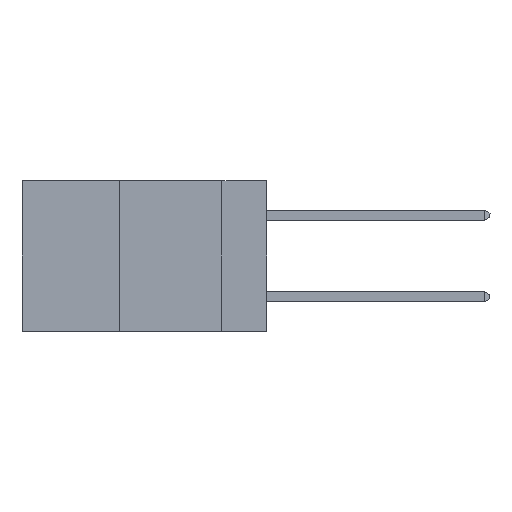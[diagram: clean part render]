
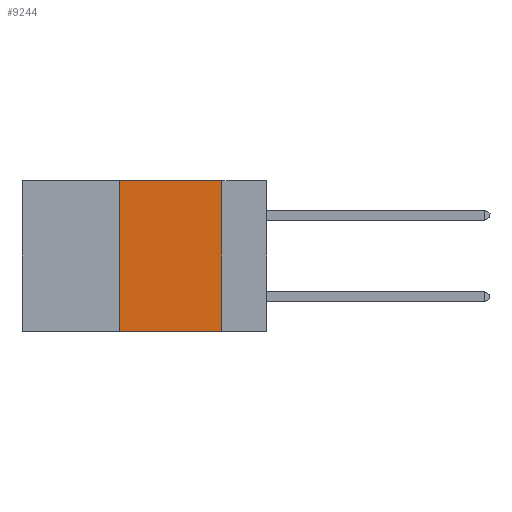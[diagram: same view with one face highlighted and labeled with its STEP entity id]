
A CAD part, left-side view. The second image highlights one B-rep face of the part: STEP entity #9244.
In plain terms, the highlighted planar face has unit normal (-1, 0, 0).
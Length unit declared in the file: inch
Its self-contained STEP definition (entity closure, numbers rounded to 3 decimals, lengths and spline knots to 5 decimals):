
#598 = CARTESIAN_POINT ( 'NONE',  ( 0., 0.36, -0.37 ) ) ;
#682 = AXIS2_PLACEMENT_3D ( 'NONE', #1730, #8000, #1774 ) ;
#913 = CARTESIAN_POINT ( 'NONE',  ( 0., 0.11, -0.37 ) ) ;
#1730 = CARTESIAN_POINT ( 'NONE',  ( 0., 0.6, 0. ) ) ;
#1774 = DIRECTION ( 'NONE',  ( 0., 0., -1. ) ) ;
#1856 = VERTEX_POINT ( 'NONE', #3562 ) ;
#2295 = LINE ( 'NONE', #10080, #4406 ) ;
#2732 = LINE ( 'NONE', #8304, #13444 ) ;
#2985 = EDGE_CURVE ( 'NONE', #7192, #11827, #3930, .T. ) ;
#3562 = CARTESIAN_POINT ( 'NONE',  ( 0., 0.36, 0. ) ) ;
#3793 = DIRECTION ( 'NONE',  ( 0., 0., -1. ) ) ;
#3861 = DIRECTION ( 'NONE',  ( 0., 0., 1. ) ) ;
#3930 = LINE ( 'NONE', #6907, #6392 ) ;
#4406 = VECTOR ( 'NONE', #3861, 39.37008 ) ;
#4591 = DIRECTION ( 'NONE',  ( 0., -1., 0. ) ) ;
#6392 = VECTOR ( 'NONE', #3793, 39.37008 ) ;
#6407 = EDGE_LOOP ( 'NONE', ( #9040, #9282, #9295, #10539 ) ) ;
#6743 = FACE_OUTER_BOUND ( 'NONE', #6407, .T. ) ;
#6863 = EDGE_CURVE ( 'NONE', #1856, #7192, #9538, .T. ) ;
#6907 = CARTESIAN_POINT ( 'NONE',  ( 0., 0.11, 0. ) ) ;
#6994 = PLANE ( 'NONE',  #682 ) ;
#7192 = VERTEX_POINT ( 'NONE', #11375 ) ;
#8000 = DIRECTION ( 'NONE',  ( 1., 0., 0. ) ) ;
#8304 = CARTESIAN_POINT ( 'NONE',  ( 0., 0.6, -0.37 ) ) ;
#9040 = ORIENTED_EDGE ( 'NONE', *, *, #2985, .F. ) ;
#9137 = VERTEX_POINT ( 'NONE', #598 ) ;
#9244 = ADVANCED_FACE ( 'NONE', ( #6743 ), #6994, .F. ) ;
#9282 = ORIENTED_EDGE ( 'NONE', *, *, #6863, .F. ) ;
#9295 = ORIENTED_EDGE ( 'NONE', *, *, #11668, .F. ) ;
#9538 = LINE ( 'NONE', #9803, #11694 ) ;
#9803 = CARTESIAN_POINT ( 'NONE',  ( 0., 0.6, 0. ) ) ;
#10080 = CARTESIAN_POINT ( 'NONE',  ( 0., 0.36, 0. ) ) ;
#10539 = ORIENTED_EDGE ( 'NONE', *, *, #13187, .T. ) ;
#11375 = CARTESIAN_POINT ( 'NONE',  ( 0., 0.11, 0. ) ) ;
#11506 = DIRECTION ( 'NONE',  ( 0., -1., 0. ) ) ;
#11668 = EDGE_CURVE ( 'NONE', #9137, #1856, #2295, .T. ) ;
#11694 = VECTOR ( 'NONE', #4591, 39.37008 ) ;
#11827 = VERTEX_POINT ( 'NONE', #913 ) ;
#13187 = EDGE_CURVE ( 'NONE', #9137, #11827, #2732, .T. ) ;
#13444 = VECTOR ( 'NONE', #11506, 39.37008 ) ;
